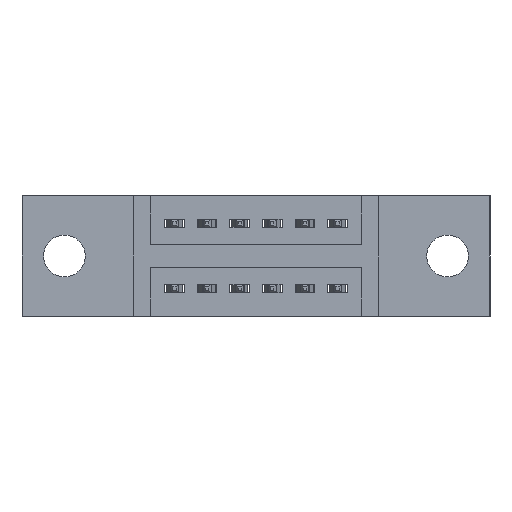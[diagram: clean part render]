
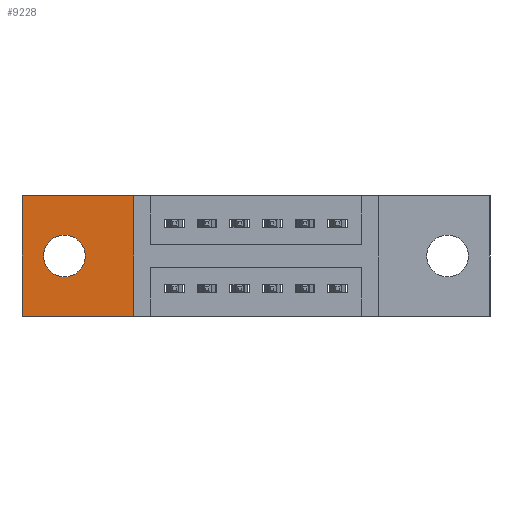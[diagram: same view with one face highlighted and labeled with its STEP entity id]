
A CAD part, front view. The second image highlights one B-rep face of the part: STEP entity #9228.
In plain terms, the highlighted planar face has unit normal (0, -1, 0).
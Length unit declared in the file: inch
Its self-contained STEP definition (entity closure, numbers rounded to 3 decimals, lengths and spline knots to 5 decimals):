
#302 = LINE ( 'NONE', #2586, #6679 ) ;
#339 = DIRECTION ( 'NONE',  ( -1., 0., 0. ) ) ;
#344 = ORIENTED_EDGE ( 'NONE', *, *, #6389, .T. ) ;
#489 = CIRCLE ( 'NONE', #4274, 0.064 ) ;
#513 = ORIENTED_EDGE ( 'NONE', *, *, #1730, .T. ) ;
#661 = DIRECTION ( 'NONE',  ( 1., 0., 0. ) ) ;
#778 = DIRECTION ( 'NONE',  ( 0., 0., -1. ) ) ;
#1190 = EDGE_CURVE ( 'NONE', #2507, #5902, #1252, .T. ) ;
#1228 = EDGE_CURVE ( 'NONE', #7892, #6238, #6435, .T. ) ;
#1252 = CIRCLE ( 'NONE', #5180, 0.064 ) ;
#1355 = LINE ( 'NONE', #5188, #9101 ) ;
#1730 = EDGE_CURVE ( 'NONE', #8823, #2519, #2302, .T. ) ;
#1893 = CARTESIAN_POINT ( 'NONE',  ( 0.13, 0.17, -0.185 ) ) ;
#1955 = VECTOR ( 'NONE', #5609, 39.37008 ) ;
#2302 = LINE ( 'NONE', #7130, #1955 ) ;
#2382 = CARTESIAN_POINT ( 'NONE',  ( 0., 0.17, -0.37 ) ) ;
#2507 = VERTEX_POINT ( 'NONE', #7852 ) ;
#2519 = VERTEX_POINT ( 'NONE', #6339 ) ;
#2586 = CARTESIAN_POINT ( 'NONE',  ( 0., 0.17, 0. ) ) ;
#2591 = DIRECTION ( 'NONE',  ( 0., 0., -1. ) ) ;
#2725 = EDGE_CURVE ( 'NONE', #2519, #7892, #1355, .T. ) ;
#2799 = ORIENTED_EDGE ( 'NONE', *, *, #1190, .F. ) ;
#3041 = PLANE ( 'NONE',  #8804 ) ;
#3103 = DIRECTION ( 'NONE',  ( 0., -1., 0. ) ) ;
#3289 = EDGE_CURVE ( 'NONE', #5902, #2507, #489, .T. ) ;
#3347 = CARTESIAN_POINT ( 'NONE',  ( 0.13, 0.17, -0.249 ) ) ;
#3401 = CARTESIAN_POINT ( 'NONE',  ( 0.13, 0.17, -0.185 ) ) ;
#3416 = DIRECTION ( 'NONE',  ( 0., 0., 1. ) ) ;
#3439 = DIRECTION ( 'NONE',  ( 0., -1., 0. ) ) ;
#4008 = CARTESIAN_POINT ( 'NONE',  ( 0., 0.17, 0. ) ) ;
#4162 = ORIENTED_EDGE ( 'NONE', *, *, #3289, .F. ) ;
#4194 = DIRECTION ( 'NONE',  ( 0., 0., -1. ) ) ;
#4274 = AXIS2_PLACEMENT_3D ( 'NONE', #1893, #8562, #2591 ) ;
#4579 = EDGE_LOOP ( 'NONE', ( #2799, #4162 ) ) ;
#4608 = FACE_OUTER_BOUND ( 'NONE', #8350, .T. ) ;
#5180 = AXIS2_PLACEMENT_3D ( 'NONE', #3401, #3439, #4194 ) ;
#5188 = CARTESIAN_POINT ( 'NONE',  ( 0., 0.17, -0.37 ) ) ;
#5194 = CARTESIAN_POINT ( 'NONE',  ( 0.3425, 0.17, 0. ) ) ;
#5609 = DIRECTION ( 'NONE',  ( 0., 0., -1. ) ) ;
#5672 = FACE_BOUND ( 'NONE', #4579, .T. ) ;
#5902 = VERTEX_POINT ( 'NONE', #3347 ) ;
#6238 = VERTEX_POINT ( 'NONE', #6863 ) ;
#6266 = CARTESIAN_POINT ( 'NONE',  ( 0.3425, 0.17, -0.37 ) ) ;
#6339 = CARTESIAN_POINT ( 'NONE',  ( 0., 0.17, -0.37 ) ) ;
#6389 = EDGE_CURVE ( 'NONE', #6238, #8823, #302, .T. ) ;
#6394 = ORIENTED_EDGE ( 'NONE', *, *, #2725, .T. ) ;
#6435 = LINE ( 'NONE', #5194, #6907 ) ;
#6679 = VECTOR ( 'NONE', #339, 39.37008 ) ;
#6863 = CARTESIAN_POINT ( 'NONE',  ( 0.3425, 0.17, 0. ) ) ;
#6907 = VECTOR ( 'NONE', #3416, 39.37008 ) ;
#7130 = CARTESIAN_POINT ( 'NONE',  ( 0., 0.17, 0. ) ) ;
#7852 = CARTESIAN_POINT ( 'NONE',  ( 0.13, 0.17, -0.121 ) ) ;
#7892 = VERTEX_POINT ( 'NONE', #6266 ) ;
#8350 = EDGE_LOOP ( 'NONE', ( #513, #6394, #8653, #344 ) ) ;
#8562 = DIRECTION ( 'NONE',  ( 0., -1., 0. ) ) ;
#8653 = ORIENTED_EDGE ( 'NONE', *, *, #1228, .T. ) ;
#8804 = AXIS2_PLACEMENT_3D ( 'NONE', #2382, #3103, #778 ) ;
#8823 = VERTEX_POINT ( 'NONE', #4008 ) ;
#9101 = VECTOR ( 'NONE', #661, 39.37008 ) ;
#9228 = ADVANCED_FACE ( 'NONE', ( #5672, #4608 ), #3041, .T. ) ;
